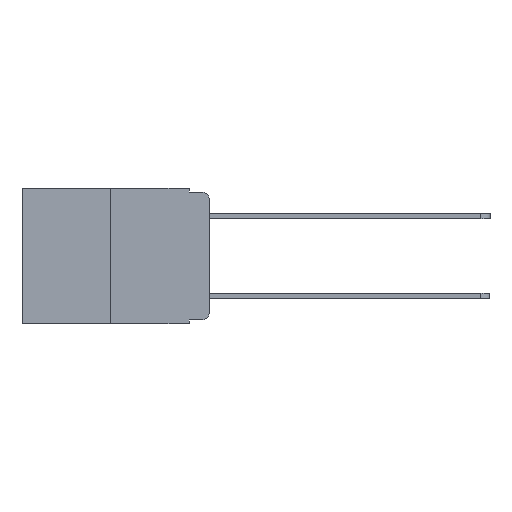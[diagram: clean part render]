
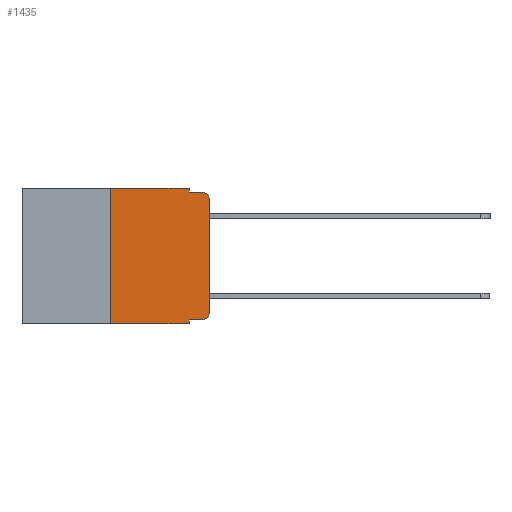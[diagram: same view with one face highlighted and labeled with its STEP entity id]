
A CAD part, left-side view. The second image highlights one B-rep face of the part: STEP entity #1435.
In plain terms, the highlighted planar face has unit normal (-1, 0, 0).
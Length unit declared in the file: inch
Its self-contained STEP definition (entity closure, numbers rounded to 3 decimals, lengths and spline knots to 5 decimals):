
#18 = CARTESIAN_POINT ( 'NONE',  ( 0., 0.25, -0.343 ) ) ;
#56 = VECTOR ( 'NONE', #6888, 39.37008 ) ;
#451 = AXIS2_PLACEMENT_3D ( 'NONE', #10503, #4371, #11488 ) ;
#471 = VERTEX_POINT ( 'NONE', #18 ) ;
#1435 = ADVANCED_FACE ( 'NONE', ( #12927 ), #11786, .F. ) ;
#1468 = ORIENTED_EDGE ( 'NONE', *, *, #7169, .T. ) ;
#2236 = VECTOR ( 'NONE', #6570, 39.37008 ) ;
#2403 = VECTOR ( 'NONE', #3147, 39.37008 ) ;
#2644 = CARTESIAN_POINT ( 'NONE',  ( 0., 0.051, -0.333 ) ) ;
#3051 = ORIENTED_EDGE ( 'NONE', *, *, #11295, .F. ) ;
#3124 = LINE ( 'NONE', #7898, #56 ) ;
#3147 = DIRECTION ( 'NONE',  ( 0., 0., -1. ) ) ;
#3265 = DIRECTION ( 'NONE',  ( 0., -1., 0. ) ) ;
#3293 = CARTESIAN_POINT ( 'NONE',  ( 0., 0.25, 0. ) ) ;
#3433 = VECTOR ( 'NONE', #6719, 39.37008 ) ;
#4120 = ORIENTED_EDGE ( 'NONE', *, *, #7839, .F. ) ;
#4317 = CARTESIAN_POINT ( 'NONE',  ( 0., 0.051, -0.333 ) ) ;
#4371 = DIRECTION ( 'NONE',  ( -1., 0., 0. ) ) ;
#4390 = AXIS2_PLACEMENT_3D ( 'NONE', #12649, #12511, #12561 ) ;
#5010 = ORIENTED_EDGE ( 'NONE', *, *, #10447, .T. ) ;
#5255 = LINE ( 'NONE', #13403, #2236 ) ;
#5420 = LINE ( 'NONE', #8508, #2403 ) ;
#5459 = CARTESIAN_POINT ( 'NONE',  ( 0., 0.051, 0. ) ) ;
#5654 = VECTOR ( 'NONE', #3265, 39.37008 ) ;
#5657 = CARTESIAN_POINT ( 'NONE',  ( 0., 0.051, 0. ) ) ;
#5793 = CIRCLE ( 'NONE', #451, 0.02 ) ;
#5928 = CARTESIAN_POINT ( 'NONE',  ( 0., 0., -0.313 ) ) ;
#5990 = LINE ( 'NONE', #9583, #5654 ) ;
#6209 = VERTEX_POINT ( 'NONE', #5928 ) ;
#6253 = CARTESIAN_POINT ( 'NONE',  ( 0., 0.051, -0.01 ) ) ;
#6287 = AXIS2_PLACEMENT_3D ( 'NONE', #12608, #10555, #11750 ) ;
#6480 = EDGE_CURVE ( 'NONE', #11304, #6209, #13190, .T. ) ;
#6570 = DIRECTION ( 'NONE',  ( 0., 0., 1. ) ) ;
#6701 = ORIENTED_EDGE ( 'NONE', *, *, #8523, .F. ) ;
#6719 = DIRECTION ( 'NONE',  ( 0., 0., -1. ) ) ;
#6888 = DIRECTION ( 'NONE',  ( 0., -1., 0. ) ) ;
#7169 = EDGE_CURVE ( 'NONE', #8199, #11304, #13010, .T. ) ;
#7342 = ORIENTED_EDGE ( 'NONE', *, *, #6480, .T. ) ;
#7766 = VERTEX_POINT ( 'NONE', #8425 ) ;
#7839 = EDGE_CURVE ( 'NONE', #8199, #8846, #5420, .T. ) ;
#7898 = CARTESIAN_POINT ( 'NONE',  ( 0., 0.473, 0. ) ) ;
#8199 = VERTEX_POINT ( 'NONE', #2644 ) ;
#8325 = VECTOR ( 'NONE', #12504, 39.37008 ) ;
#8425 = CARTESIAN_POINT ( 'NONE',  ( 0., 0.25, 0. ) ) ;
#8508 = CARTESIAN_POINT ( 'NONE',  ( 0., 0.051, 0. ) ) ;
#8523 = EDGE_CURVE ( 'NONE', #471, #7766, #10886, .T. ) ;
#8688 = EDGE_CURVE ( 'NONE', #471, #8846, #12547, .T. ) ;
#8846 = VERTEX_POINT ( 'NONE', #11062 ) ;
#8890 = CARTESIAN_POINT ( 'NONE',  ( 0., 0.473, -0.343 ) ) ;
#9049 = VERTEX_POINT ( 'NONE', #5459 ) ;
#9177 = EDGE_CURVE ( 'NONE', #9049, #10279, #11648, .T. ) ;
#9253 = CARTESIAN_POINT ( 'NONE',  ( 0., 0., -0.03 ) ) ;
#9497 = CARTESIAN_POINT ( 'NONE',  ( 0., 0.02, -0.01 ) ) ;
#9583 = CARTESIAN_POINT ( 'NONE',  ( 0., 0.051, -0.01 ) ) ;
#9693 = VECTOR ( 'NONE', #9855, 39.37008 ) ;
#9757 = VERTEX_POINT ( 'NONE', #9497 ) ;
#9826 = EDGE_CURVE ( 'NONE', #10279, #9757, #5990, .T. ) ;
#9855 = DIRECTION ( 'NONE',  ( 0., -1., 0. ) ) ;
#9865 = CARTESIAN_POINT ( 'NONE',  ( 0., 0.02, -0.333 ) ) ;
#10279 = VERTEX_POINT ( 'NONE', #6253 ) ;
#10447 = EDGE_CURVE ( 'NONE', #12996, #9757, #5793, .T. ) ;
#10448 = VECTOR ( 'NONE', #13361, 39.37008 ) ;
#10503 = CARTESIAN_POINT ( 'NONE',  ( 0., 0.02, -0.03 ) ) ;
#10555 = DIRECTION ( 'NONE',  ( -1., 0., 0. ) ) ;
#10886 = LINE ( 'NONE', #3293, #8325 ) ;
#11062 = CARTESIAN_POINT ( 'NONE',  ( 0., 0.051, -0.343 ) ) ;
#11101 = EDGE_CURVE ( 'NONE', #6209, #12996, #5255, .T. ) ;
#11157 = EDGE_LOOP ( 'NONE', ( #12372, #5010, #12952, #13579, #3051, #6701, #11934, #4120, #1468, #7342 ) ) ;
#11295 = EDGE_CURVE ( 'NONE', #7766, #9049, #3124, .T. ) ;
#11304 = VERTEX_POINT ( 'NONE', #9865 ) ;
#11488 = DIRECTION ( 'NONE',  ( 0., 0., -1. ) ) ;
#11648 = LINE ( 'NONE', #5657, #3433 ) ;
#11750 = DIRECTION ( 'NONE',  ( 0., 0., -1. ) ) ;
#11786 = PLANE ( 'NONE',  #4390 ) ;
#11934 = ORIENTED_EDGE ( 'NONE', *, *, #8688, .T. ) ;
#12372 = ORIENTED_EDGE ( 'NONE', *, *, #11101, .T. ) ;
#12504 = DIRECTION ( 'NONE',  ( 0., 0., 1. ) ) ;
#12511 = DIRECTION ( 'NONE',  ( 1., 0., 0. ) ) ;
#12547 = LINE ( 'NONE', #8890, #9693 ) ;
#12561 = DIRECTION ( 'NONE',  ( 0., 0., -1. ) ) ;
#12608 = CARTESIAN_POINT ( 'NONE',  ( 0., 0.02, -0.313 ) ) ;
#12649 = CARTESIAN_POINT ( 'NONE',  ( 0., 0.473, 0. ) ) ;
#12927 = FACE_OUTER_BOUND ( 'NONE', #11157, .T. ) ;
#12952 = ORIENTED_EDGE ( 'NONE', *, *, #9826, .F. ) ;
#12996 = VERTEX_POINT ( 'NONE', #9253 ) ;
#13010 = LINE ( 'NONE', #4317, #10448 ) ;
#13190 = CIRCLE ( 'NONE', #6287, 0.02 ) ;
#13361 = DIRECTION ( 'NONE',  ( 0., -1., 0. ) ) ;
#13403 = CARTESIAN_POINT ( 'NONE',  ( 0., 0., 0. ) ) ;
#13579 = ORIENTED_EDGE ( 'NONE', *, *, #9177, .F. ) ;
